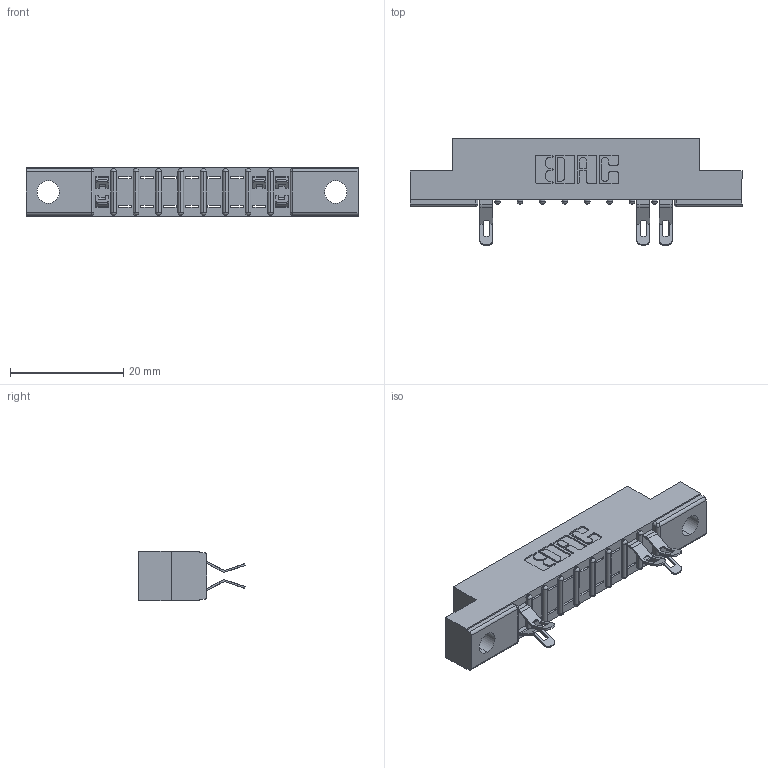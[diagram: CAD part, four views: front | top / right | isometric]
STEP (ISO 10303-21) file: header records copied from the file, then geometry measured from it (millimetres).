
FILE_DESCRIPTION (( 'STEP AP203' ), '1' );
FILE_NAME ('307-018-555-202.STEP', '2018-08-03T23:28:45', ( '' ), ( '' ), 'SwSTEP 2.0', 'SolidWorks 2016', '' );
FILE_SCHEMA (( 'CONFIG_CONTROL_DESIGN' ));
Length unit declared in the file: inch
Products named in the file (3): 307 Part_.128 Dia Mounting Holes; 307-290-001_555; 307-018-555-202
Assembly tree (6 placements, depth 2):
  307-018-555-202
    307 Part_.128 Dia Mounting Holes
    307-290-001_555  x5
Bounding box: 58.67 x 18.75 x 8.71 mm (x, y, z)
Volume: 3598.1 mm3; surface area: 4612.3 mm2
Topology: 6 solids, 6 shells, 563 faces, 1644 edges, 1060 vertices
Faces by surface type: plane 318, cylinder 225, sphere 20
Entity records: 12195 total; most frequent: CARTESIAN_POINT 2064, ORIENTED_EDGE 2056, DIRECTION 2030, EDGE_CURVE 1028, VECTOR 762, LINE 762, VERTEX_POINT 668, AXIS2_PLACEMENT_3D 634
